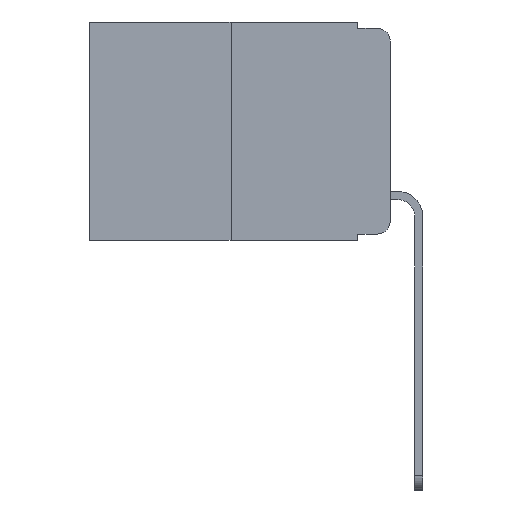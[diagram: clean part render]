
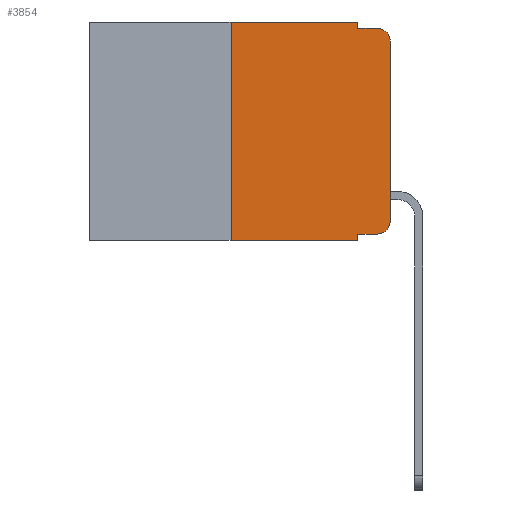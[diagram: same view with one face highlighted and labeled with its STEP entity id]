
A CAD part, left-side view. The second image highlights one B-rep face of the part: STEP entity #3854.
In plain terms, the highlighted planar face has unit normal (-1, 0, 0).
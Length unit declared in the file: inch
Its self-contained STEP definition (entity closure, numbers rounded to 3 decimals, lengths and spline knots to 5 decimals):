
#298 = ORIENTED_EDGE ( 'NONE', *, *, #3022, .F. ) ;
#498 = ORIENTED_EDGE ( 'NONE', *, *, #6635, .T. ) ;
#527 = ORIENTED_EDGE ( 'NONE', *, *, #6501, .F. ) ;
#560 = LINE ( 'NONE', #8906, #6068 ) ;
#787 = EDGE_CURVE ( 'NONE', #10218, #9792, #12097, .T. ) ;
#852 = CIRCLE ( 'NONE', #4855, 0.02 ) ;
#863 = CARTESIAN_POINT ( 'NONE',  ( 0., 0.051, -0.343 ) ) ;
#1699 = VECTOR ( 'NONE', #12252, 39.37008 ) ;
#1783 = VERTEX_POINT ( 'NONE', #11560 ) ;
#1828 = CARTESIAN_POINT ( 'NONE',  ( 0., 0.051, -0.01 ) ) ;
#1979 = VERTEX_POINT ( 'NONE', #8377 ) ;
#2064 = LINE ( 'NONE', #5241, #11660 ) ;
#2223 = VERTEX_POINT ( 'NONE', #4747 ) ;
#2778 = ORIENTED_EDGE ( 'NONE', *, *, #6485, .F. ) ;
#2888 = VERTEX_POINT ( 'NONE', #11116 ) ;
#3022 = EDGE_CURVE ( 'NONE', #2223, #3207, #560, .T. ) ;
#3184 = ORIENTED_EDGE ( 'NONE', *, *, #787, .T. ) ;
#3190 = EDGE_LOOP ( 'NONE', ( #8576, #8843, #9119, #2778, #298, #527, #3184, #10649, #498, #12260 ) ) ;
#3207 = VERTEX_POINT ( 'NONE', #3422 ) ;
#3422 = CARTESIAN_POINT ( 'NONE',  ( 0., 0.051, 0. ) ) ;
#3430 = LINE ( 'NONE', #9338, #10687 ) ;
#3690 = CARTESIAN_POINT ( 'NONE',  ( 0., 0.051, -0.333 ) ) ;
#3854 = ADVANCED_FACE ( 'NONE', ( #7446 ), #11146, .F. ) ;
#4067 = CARTESIAN_POINT ( 'NONE',  ( 0., 0.02, -0.03 ) ) ;
#4747 = CARTESIAN_POINT ( 'NONE',  ( 0., 0.25, 0. ) ) ;
#4768 = CARTESIAN_POINT ( 'NONE',  ( 0., 0.02, -0.313 ) ) ;
#4818 = LINE ( 'NONE', #6194, #1699 ) ;
#4836 = CARTESIAN_POINT ( 'NONE',  ( 0., 0.473, 0. ) ) ;
#4855 = AXIS2_PLACEMENT_3D ( 'NONE', #4768, #11095, #5782 ) ;
#5120 = DIRECTION ( 'NONE',  ( 0., 0., -1. ) ) ;
#5168 = AXIS2_PLACEMENT_3D ( 'NONE', #4067, #10600, #5120 ) ;
#5241 = CARTESIAN_POINT ( 'NONE',  ( 0., 0.25, 0. ) ) ;
#5257 = VECTOR ( 'NONE', #12401, 39.37008 ) ;
#5436 = CIRCLE ( 'NONE', #5168, 0.02 ) ;
#5782 = DIRECTION ( 'NONE',  ( 0., 0., -1. ) ) ;
#6068 = VECTOR ( 'NONE', #7896, 39.37008 ) ;
#6183 = EDGE_CURVE ( 'NONE', #1979, #2888, #3430, .T. ) ;
#6194 = CARTESIAN_POINT ( 'NONE',  ( 0., 0.051, 0. ) ) ;
#6278 = CARTESIAN_POINT ( 'NONE',  ( 0., 0.051, 0. ) ) ;
#6412 = EDGE_CURVE ( 'NONE', #2888, #1783, #5436, .T. ) ;
#6466 = EDGE_CURVE ( 'NONE', #11457, #1783, #7668, .T. ) ;
#6485 = EDGE_CURVE ( 'NONE', #3207, #11457, #4818, .T. ) ;
#6501 = EDGE_CURVE ( 'NONE', #10218, #2223, #2064, .T. ) ;
#6543 = EDGE_CURVE ( 'NONE', #11082, #9792, #7083, .T. ) ;
#6635 = EDGE_CURVE ( 'NONE', #11082, #9953, #12282, .T. ) ;
#6787 = DIRECTION ( 'NONE',  ( 0., 0., -1. ) ) ;
#6801 = EDGE_CURVE ( 'NONE', #9953, #1979, #852, .T. ) ;
#7083 = LINE ( 'NONE', #6278, #9177 ) ;
#7105 = DIRECTION ( 'NONE',  ( 0., -1., 0. ) ) ;
#7341 = CARTESIAN_POINT ( 'NONE',  ( 0., 0.051, -0.333 ) ) ;
#7370 = VECTOR ( 'NONE', #7105, 39.37008 ) ;
#7446 = FACE_OUTER_BOUND ( 'NONE', #3190, .T. ) ;
#7522 = CARTESIAN_POINT ( 'NONE',  ( 0., 0.02, -0.333 ) ) ;
#7567 = DIRECTION ( 'NONE',  ( 0., 0., 1. ) ) ;
#7668 = LINE ( 'NONE', #8905, #7370 ) ;
#7834 = CARTESIAN_POINT ( 'NONE',  ( 0., 0.25, -0.343 ) ) ;
#7896 = DIRECTION ( 'NONE',  ( 0., -1., 0. ) ) ;
#8004 = AXIS2_PLACEMENT_3D ( 'NONE', #4836, #11948, #6787 ) ;
#8377 = CARTESIAN_POINT ( 'NONE',  ( 0., 0., -0.313 ) ) ;
#8576 = ORIENTED_EDGE ( 'NONE', *, *, #6183, .T. ) ;
#8843 = ORIENTED_EDGE ( 'NONE', *, *, #6412, .T. ) ;
#8905 = CARTESIAN_POINT ( 'NONE',  ( 0., 0.051, -0.01 ) ) ;
#8906 = CARTESIAN_POINT ( 'NONE',  ( 0., 0.473, 0. ) ) ;
#9119 = ORIENTED_EDGE ( 'NONE', *, *, #6466, .F. ) ;
#9165 = CARTESIAN_POINT ( 'NONE',  ( 0., 0.473, -0.343 ) ) ;
#9177 = VECTOR ( 'NONE', #10733, 39.37008 ) ;
#9338 = CARTESIAN_POINT ( 'NONE',  ( 0., 0., 0. ) ) ;
#9792 = VERTEX_POINT ( 'NONE', #863 ) ;
#9953 = VERTEX_POINT ( 'NONE', #7522 ) ;
#10114 = DIRECTION ( 'NONE',  ( 0., -1., 0. ) ) ;
#10218 = VERTEX_POINT ( 'NONE', #7834 ) ;
#10600 = DIRECTION ( 'NONE',  ( -1., 0., 0. ) ) ;
#10649 = ORIENTED_EDGE ( 'NONE', *, *, #6543, .F. ) ;
#10687 = VECTOR ( 'NONE', #7567, 39.37008 ) ;
#10696 = DIRECTION ( 'NONE',  ( 0., 0., 1. ) ) ;
#10733 = DIRECTION ( 'NONE',  ( 0., 0., -1. ) ) ;
#11082 = VERTEX_POINT ( 'NONE', #3690 ) ;
#11095 = DIRECTION ( 'NONE',  ( -1., 0., 0. ) ) ;
#11116 = CARTESIAN_POINT ( 'NONE',  ( 0., 0., -0.03 ) ) ;
#11146 = PLANE ( 'NONE',  #8004 ) ;
#11457 = VERTEX_POINT ( 'NONE', #1828 ) ;
#11560 = CARTESIAN_POINT ( 'NONE',  ( 0., 0.02, -0.01 ) ) ;
#11660 = VECTOR ( 'NONE', #10696, 39.37008 ) ;
#11846 = VECTOR ( 'NONE', #10114, 39.37008 ) ;
#11948 = DIRECTION ( 'NONE',  ( 1., 0., 0. ) ) ;
#12097 = LINE ( 'NONE', #9165, #11846 ) ;
#12252 = DIRECTION ( 'NONE',  ( 0., 0., -1. ) ) ;
#12260 = ORIENTED_EDGE ( 'NONE', *, *, #6801, .T. ) ;
#12282 = LINE ( 'NONE', #7341, #5257 ) ;
#12401 = DIRECTION ( 'NONE',  ( 0., -1., 0. ) ) ;
